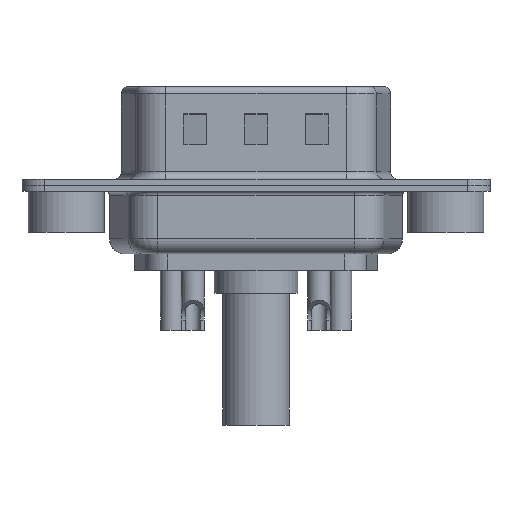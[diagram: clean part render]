
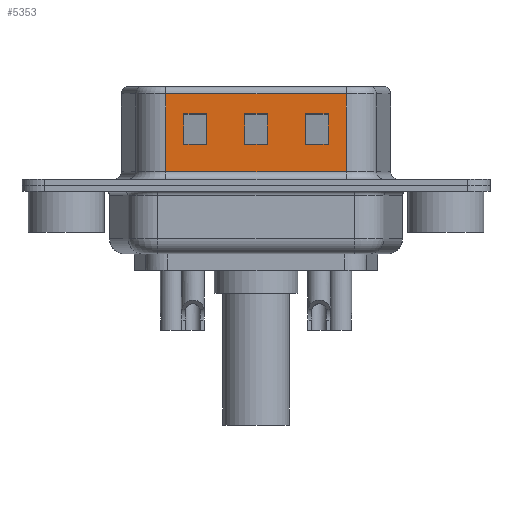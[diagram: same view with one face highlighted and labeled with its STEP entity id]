
A CAD part, front view. The second image highlights one B-rep face of the part: STEP entity #5353.
In plain terms, the highlighted planar face has unit normal (0, -1, 0).
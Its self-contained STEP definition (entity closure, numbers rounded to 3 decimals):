
#143 = VERTEX_POINT ( 'NONE', #9397 ) ;
#209 = VECTOR ( 'NONE', #862, 1000. ) ;
#414 = CARTESIAN_POINT ( 'NONE',  ( 17.25, -4.58, 2.705 ) ) ;
#481 = VERTEX_POINT ( 'NONE', #12603 ) ;
#670 = CARTESIAN_POINT ( 'NONE',  ( 17.25, -4.58, 4.705 ) ) ;
#762 = DIRECTION ( 'NONE',  ( -1., 0., 0. ) ) ;
#774 = CARTESIAN_POINT ( 'NONE',  ( 6.55, -4.58, 6.52 ) ) ;
#815 = VERTEX_POINT ( 'NONE', #8843 ) ;
#834 = LINE ( 'NONE', #13577, #9006 ) ;
#862 = DIRECTION ( 'NONE',  ( 0., 0., -1. ) ) ;
#873 = VERTEX_POINT ( 'NONE', #670 ) ;
#1058 = CARTESIAN_POINT ( 'NONE',  ( 9.25, -4.58, 2.705 ) ) ;
#1089 = LINE ( 'NONE', #12455, #6333 ) ;
#1096 = EDGE_CURVE ( 'NONE', #9555, #8734, #6177, .T. ) ;
#1367 = LINE ( 'NONE', #8594, #12757 ) ;
#1393 = VERTEX_POINT ( 'NONE', #6835 ) ;
#1466 = VECTOR ( 'NONE', #2901, 1000. ) ;
#1479 = VERTEX_POINT ( 'NONE', #14337 ) ;
#1581 = CARTESIAN_POINT ( 'NONE',  ( 18.45, -4.58, 2.705 ) ) ;
#1585 = DIRECTION ( 'NONE',  ( -1., 0., 0. ) ) ;
#1631 = VERTEX_POINT ( 'NONE', #2811 ) ;
#1725 = ORIENTED_EDGE ( 'NONE', *, *, #5665, .T. ) ;
#2062 = VERTEX_POINT ( 'NONE', #8036 ) ;
#2068 = VECTOR ( 'NONE', #12585, 1000. ) ;
#2107 = DIRECTION ( 'NONE',  ( 1., 0., 0. ) ) ;
#2152 = CARTESIAN_POINT ( 'NONE',  ( 18.45, -4.58, 0.9 ) ) ;
#2166 = CARTESIAN_POINT ( 'NONE',  ( 15.75, -4.58, 4.705 ) ) ;
#2201 = EDGE_CURVE ( 'NONE', #8734, #4332, #5834, .T. ) ;
#2452 = DIRECTION ( 'NONE',  ( 1., 0., 0. ) ) ;
#2614 = ORIENTED_EDGE ( 'NONE', *, *, #1096, .T. ) ;
#2635 = ORIENTED_EDGE ( 'NONE', *, *, #11764, .T. ) ;
#2811 = CARTESIAN_POINT ( 'NONE',  ( 11.75, -4.58, 4.705 ) ) ;
#2901 = DIRECTION ( 'NONE',  ( 1., 0., 0. ) ) ;
#2959 = EDGE_CURVE ( 'NONE', #1393, #1631, #9602, .T. ) ;
#3003 = ORIENTED_EDGE ( 'NONE', *, *, #6605, .T. ) ;
#3040 = CARTESIAN_POINT ( 'NONE',  ( 11.75, -4.58, 6.52 ) ) ;
#3079 = LINE ( 'NONE', #1581, #5972 ) ;
#3220 = LINE ( 'NONE', #4001, #11617 ) ;
#3234 = DIRECTION ( 'NONE',  ( 0., 0., 1. ) ) ;
#3392 = FACE_OUTER_BOUND ( 'NONE', #13849, .T. ) ;
#3464 = ORIENTED_EDGE ( 'NONE', *, *, #5147, .T. ) ;
#3591 = CARTESIAN_POINT ( 'NONE',  ( 18.45, -4.58, 4.705 ) ) ;
#3711 = EDGE_CURVE ( 'NONE', #4983, #1393, #3079, .T. ) ;
#3712 = PLANE ( 'NONE',  #5617 ) ;
#3746 = FACE_BOUND ( 'NONE', #10033, .T. ) ;
#3753 = ORIENTED_EDGE ( 'NONE', *, *, #10308, .T. ) ;
#4001 = CARTESIAN_POINT ( 'NONE',  ( 13.25, -4.58, 6.52 ) ) ;
#4037 = CARTESIAN_POINT ( 'NONE',  ( 13.25, -4.58, 2.705 ) ) ;
#4126 = VECTOR ( 'NONE', #5711, 1000. ) ;
#4324 = LINE ( 'NONE', #4919, #2068 ) ;
#4332 = VERTEX_POINT ( 'NONE', #2152 ) ;
#4411 = CARTESIAN_POINT ( 'NONE',  ( 7.75, -4.58, 4.705 ) ) ;
#4798 = DIRECTION ( 'NONE',  ( -1., 0., 0. ) ) ;
#4919 = CARTESIAN_POINT ( 'NONE',  ( 9.25, -4.58, 6.52 ) ) ;
#4966 = ORIENTED_EDGE ( 'NONE', *, *, #2959, .T. ) ;
#4983 = VERTEX_POINT ( 'NONE', #4037 ) ;
#5118 = ORIENTED_EDGE ( 'NONE', *, *, #3711, .T. ) ;
#5147 = EDGE_CURVE ( 'NONE', #815, #4983, #3220, .T. ) ;
#5210 = VECTOR ( 'NONE', #14354, 1000. ) ;
#5303 = VECTOR ( 'NONE', #12742, 1000. ) ;
#5332 = ORIENTED_EDGE ( 'NONE', *, *, #12485, .T. ) ;
#5353 = ADVANCED_FACE ( 'NONE', ( #6288, #12118, #3746, #3392 ), #3712, .F. ) ;
#5361 = EDGE_LOOP ( 'NONE', ( #7676, #5332, #2635, #7135 ) ) ;
#5617 = AXIS2_PLACEMENT_3D ( 'NONE', #11458, #6984, #3234 ) ;
#5665 = EDGE_CURVE ( 'NONE', #481, #9555, #6444, .T. ) ;
#5711 = DIRECTION ( 'NONE',  ( 0., 0., 1. ) ) ;
#5834 = LINE ( 'NONE', #13764, #11351 ) ;
#5867 = EDGE_CURVE ( 'NONE', #1631, #815, #13498, .T. ) ;
#5972 = VECTOR ( 'NONE', #1585, 1000. ) ;
#6177 = LINE ( 'NONE', #774, #209 ) ;
#6288 = FACE_BOUND ( 'NONE', #5361, .T. ) ;
#6296 = VERTEX_POINT ( 'NONE', #1058 ) ;
#6333 = VECTOR ( 'NONE', #4798, 1000. ) ;
#6340 = VERTEX_POINT ( 'NONE', #2166 ) ;
#6444 = LINE ( 'NONE', #10436, #9033 ) ;
#6445 = DIRECTION ( 'NONE',  ( 0., 0., -1. ) ) ;
#6605 = EDGE_CURVE ( 'NONE', #6340, #873, #834, .T. ) ;
#6668 = CARTESIAN_POINT ( 'NONE',  ( 22.45, -4.58, 2.705 ) ) ;
#6757 = ORIENTED_EDGE ( 'NONE', *, *, #8818, .T. ) ;
#6827 = DIRECTION ( 'NONE',  ( 0., 0., -1. ) ) ;
#6835 = CARTESIAN_POINT ( 'NONE',  ( 11.75, -4.58, 2.705 ) ) ;
#6963 = VECTOR ( 'NONE', #2452, 1000. ) ;
#6984 = DIRECTION ( 'NONE',  ( 0., 1., 0. ) ) ;
#7090 = DIRECTION ( 'NONE',  ( 0., 0., 1. ) ) ;
#7135 = ORIENTED_EDGE ( 'NONE', *, *, #11038, .T. ) ;
#7227 = VECTOR ( 'NONE', #12094, 1000. ) ;
#7341 = EDGE_CURVE ( 'NONE', #1479, #6340, #1367, .T. ) ;
#7676 = ORIENTED_EDGE ( 'NONE', *, *, #13238, .T. ) ;
#7759 = ORIENTED_EDGE ( 'NONE', *, *, #7341, .T. ) ;
#8036 = CARTESIAN_POINT ( 'NONE',  ( 9.25, -4.58, 4.705 ) ) ;
#8117 = LINE ( 'NONE', #6668, #5210 ) ;
#8212 = LINE ( 'NONE', #11639, #5303 ) ;
#8594 = CARTESIAN_POINT ( 'NONE',  ( 15.75, -4.58, 6.52 ) ) ;
#8734 = VERTEX_POINT ( 'NONE', #14211 ) ;
#8789 = CARTESIAN_POINT ( 'NONE',  ( 17.25, -4.58, 6.52 ) ) ;
#8818 = EDGE_CURVE ( 'NONE', #9114, #1479, #8117, .T. ) ;
#8843 = CARTESIAN_POINT ( 'NONE',  ( 13.25, -4.58, 4.705 ) ) ;
#9006 = VECTOR ( 'NONE', #14344, 1000. ) ;
#9033 = VECTOR ( 'NONE', #762, 1000. ) ;
#9114 = VERTEX_POINT ( 'NONE', #414 ) ;
#9397 = CARTESIAN_POINT ( 'NONE',  ( 7.75, -4.58, 2.705 ) ) ;
#9555 = VERTEX_POINT ( 'NONE', #10795 ) ;
#9602 = LINE ( 'NONE', #3040, #4126 ) ;
#9655 = VERTEX_POINT ( 'NONE', #4411 ) ;
#9846 = EDGE_LOOP ( 'NONE', ( #3753, #6757, #7759, #3003 ) ) ;
#9962 = LINE ( 'NONE', #13869, #1466 ) ;
#10033 = EDGE_LOOP ( 'NONE', ( #11193, #3464, #5118, #4966 ) ) ;
#10308 = EDGE_CURVE ( 'NONE', #873, #9114, #13060, .T. ) ;
#10436 = CARTESIAN_POINT ( 'NONE',  ( 18.45, -4.58, 6.02 ) ) ;
#10550 = ORIENTED_EDGE ( 'NONE', *, *, #2201, .T. ) ;
#10795 = CARTESIAN_POINT ( 'NONE',  ( 6.55, -4.58, 6.02 ) ) ;
#11038 = EDGE_CURVE ( 'NONE', #9655, #2062, #9962, .T. ) ;
#11193 = ORIENTED_EDGE ( 'NONE', *, *, #5867, .T. ) ;
#11351 = VECTOR ( 'NONE', #2107, 1000. ) ;
#11458 = CARTESIAN_POINT ( 'NONE',  ( 18.45, -4.58, 6.52 ) ) ;
#11617 = VECTOR ( 'NONE', #6827, 1000. ) ;
#11639 = CARTESIAN_POINT ( 'NONE',  ( 7.75, -4.58, 6.52 ) ) ;
#11764 = EDGE_CURVE ( 'NONE', #143, #9655, #8212, .T. ) ;
#11953 = EDGE_CURVE ( 'NONE', #481, #4332, #12864, .T. ) ;
#12094 = DIRECTION ( 'NONE',  ( 0., 0., -1. ) ) ;
#12095 = ORIENTED_EDGE ( 'NONE', *, *, #11953, .F. ) ;
#12118 = FACE_BOUND ( 'NONE', #9846, .T. ) ;
#12455 = CARTESIAN_POINT ( 'NONE',  ( 14.45, -4.58, 2.705 ) ) ;
#12485 = EDGE_CURVE ( 'NONE', #6296, #143, #1089, .T. ) ;
#12514 = VECTOR ( 'NONE', #6445, 1000. ) ;
#12585 = DIRECTION ( 'NONE',  ( 0., 0., -1. ) ) ;
#12603 = CARTESIAN_POINT ( 'NONE',  ( 18.45, -4.58, 6.02 ) ) ;
#12742 = DIRECTION ( 'NONE',  ( 0., 0., 1. ) ) ;
#12757 = VECTOR ( 'NONE', #7090, 1000. ) ;
#12864 = LINE ( 'NONE', #14137, #12514 ) ;
#13060 = LINE ( 'NONE', #8789, #7227 ) ;
#13238 = EDGE_CURVE ( 'NONE', #2062, #6296, #4324, .T. ) ;
#13498 = LINE ( 'NONE', #3591, #6963 ) ;
#13577 = CARTESIAN_POINT ( 'NONE',  ( 22.45, -4.58, 4.705 ) ) ;
#13764 = CARTESIAN_POINT ( 'NONE',  ( 18.45, -4.58, 0.9 ) ) ;
#13849 = EDGE_LOOP ( 'NONE', ( #12095, #1725, #2614, #10550 ) ) ;
#13869 = CARTESIAN_POINT ( 'NONE',  ( 14.45, -4.58, 4.705 ) ) ;
#14137 = CARTESIAN_POINT ( 'NONE',  ( 18.45, -4.58, 6.52 ) ) ;
#14211 = CARTESIAN_POINT ( 'NONE',  ( 6.55, -4.58, 0.9 ) ) ;
#14337 = CARTESIAN_POINT ( 'NONE',  ( 15.75, -4.58, 2.705 ) ) ;
#14344 = DIRECTION ( 'NONE',  ( 1., 0., 0. ) ) ;
#14354 = DIRECTION ( 'NONE',  ( -1., 0., 0. ) ) ;
